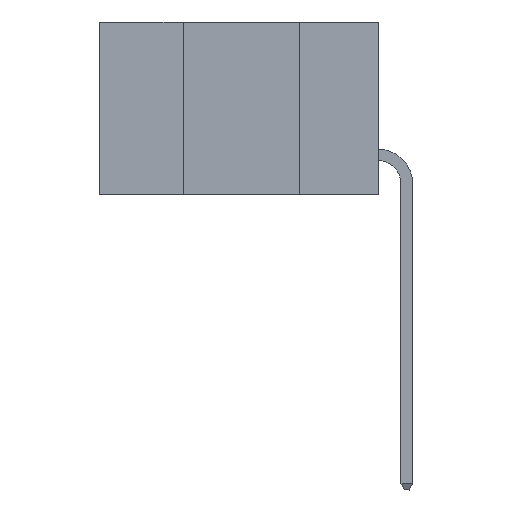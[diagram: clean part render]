
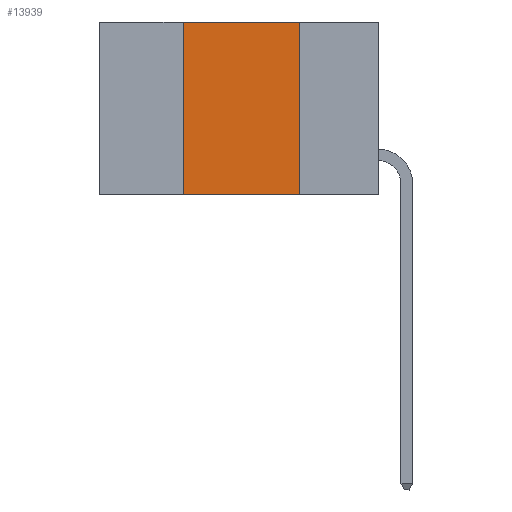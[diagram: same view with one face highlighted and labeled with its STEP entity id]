
A CAD part, left-side view. The second image highlights one B-rep face of the part: STEP entity #13939.
In plain terms, the highlighted planar face has unit normal (-1, 0, 0).
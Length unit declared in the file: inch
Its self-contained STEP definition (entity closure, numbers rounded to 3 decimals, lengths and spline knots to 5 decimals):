
#46 = EDGE_CURVE ( 'NONE', #6510, #11081, #6190, .T. ) ;
#145 = VECTOR ( 'NONE', #456, 39.37008 ) ;
#456 = DIRECTION ( 'NONE',  ( 0., -1., 0. ) ) ;
#1044 = LINE ( 'NONE', #6834, #18812 ) ;
#1834 = ORIENTED_EDGE ( 'NONE', *, *, #4193, .F. ) ;
#1876 = VERTEX_POINT ( 'NONE', #11130 ) ;
#1895 = CARTESIAN_POINT ( 'NONE',  ( 0., 0.17, -0.37 ) ) ;
#2497 = FACE_OUTER_BOUND ( 'NONE', #13242, .T. ) ;
#3179 = LINE ( 'NONE', #9277, #145 ) ;
#4193 = EDGE_CURVE ( 'NONE', #1876, #10598, #1044, .T. ) ;
#6116 = VECTOR ( 'NONE', #16016, 39.37008 ) ;
#6190 = LINE ( 'NONE', #9607, #19161 ) ;
#6510 = VERTEX_POINT ( 'NONE', #13601 ) ;
#6726 = LINE ( 'NONE', #9849, #6116 ) ;
#6834 = CARTESIAN_POINT ( 'NONE',  ( 0., 0.17, -0.37 ) ) ;
#8051 = ORIENTED_EDGE ( 'NONE', *, *, #12856, .T. ) ;
#8593 = CARTESIAN_POINT ( 'NONE',  ( 0., 0.6, 0. ) ) ;
#9051 = ORIENTED_EDGE ( 'NONE', *, *, #46, .F. ) ;
#9277 = CARTESIAN_POINT ( 'NONE',  ( 0., 0.6, 0. ) ) ;
#9607 = CARTESIAN_POINT ( 'NONE',  ( 0., 0.42, -0.37 ) ) ;
#9849 = CARTESIAN_POINT ( 'NONE',  ( 0., 0.6, -0.37 ) ) ;
#10598 = VERTEX_POINT ( 'NONE', #1895 ) ;
#11081 = VERTEX_POINT ( 'NONE', #17231 ) ;
#11130 = CARTESIAN_POINT ( 'NONE',  ( 0., 0.17, 0. ) ) ;
#11711 = DIRECTION ( 'NONE',  ( 1., 0., 0. ) ) ;
#12266 = AXIS2_PLACEMENT_3D ( 'NONE', #8593, #11711, #17851 ) ;
#12856 = EDGE_CURVE ( 'NONE', #6510, #10598, #6726, .T. ) ;
#13195 = DIRECTION ( 'NONE',  ( 0., 0., -1. ) ) ;
#13242 = EDGE_LOOP ( 'NONE', ( #1834, #17445, #9051, #8051 ) ) ;
#13601 = CARTESIAN_POINT ( 'NONE',  ( 0., 0.42, -0.37 ) ) ;
#13939 = ADVANCED_FACE ( 'NONE', ( #2497 ), #16546, .F. ) ;
#15772 = DIRECTION ( 'NONE',  ( 0., 0., 1. ) ) ;
#16016 = DIRECTION ( 'NONE',  ( 0., -1., 0. ) ) ;
#16546 = PLANE ( 'NONE',  #12266 ) ;
#16694 = EDGE_CURVE ( 'NONE', #11081, #1876, #3179, .T. ) ;
#17231 = CARTESIAN_POINT ( 'NONE',  ( 0., 0.42, 0. ) ) ;
#17445 = ORIENTED_EDGE ( 'NONE', *, *, #16694, .F. ) ;
#17851 = DIRECTION ( 'NONE',  ( 0., 0., -1. ) ) ;
#18812 = VECTOR ( 'NONE', #13195, 39.37008 ) ;
#19161 = VECTOR ( 'NONE', #15772, 39.37008 ) ;
